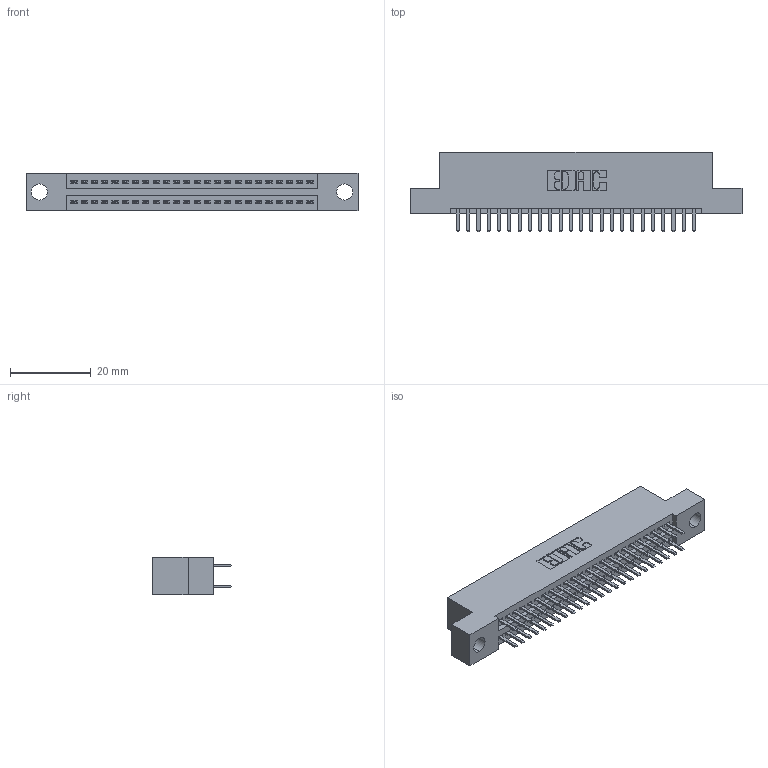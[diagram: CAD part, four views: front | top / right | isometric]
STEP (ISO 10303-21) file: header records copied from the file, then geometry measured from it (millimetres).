
FILE_DESCRIPTION (( 'STEP AP203' ), '1' );
FILE_NAME ('345-048-520-204.STEP', '2021-05-20T02:39:06', ( '' ), ( '' ), 'SwSTEP 2.0', 'SolidWorks 2020', '' );
FILE_SCHEMA (( 'CONFIG_CONTROL_DESIGN' ));
Length unit declared in the file: inch
Products named in the file (3): 345-292-001_345-293-120; 345-048-520-204; 345 Part_Flush Mounting Lugs - 0.156 Dia-TI
Assembly tree (49 placements, depth 2):
  345-048-520-204
    345 Part_Flush Mounting Lugs - 0.156 Dia-TI
    345-292-001_345-293-120  x48
Bounding box: 82.17 x 19.68 x 9.4 mm (x, y, z)
Volume: 7687.8 mm3; surface area: 10822 mm2
Topology: 49 solids, 49 shells, 2732 faces, 7913 edges, 5146 vertices
Faces by surface type: plane 1774, cylinder 958
Entity records: 21787 total; most frequent: CARTESIAN_POINT 3686, ORIENTED_EDGE 3606, DIRECTION 3259, EDGE_CURVE 1803, VECTOR 1571, LINE 1571, VERTEX_POINT 1198, AXIS2_PLACEMENT_3D 844
